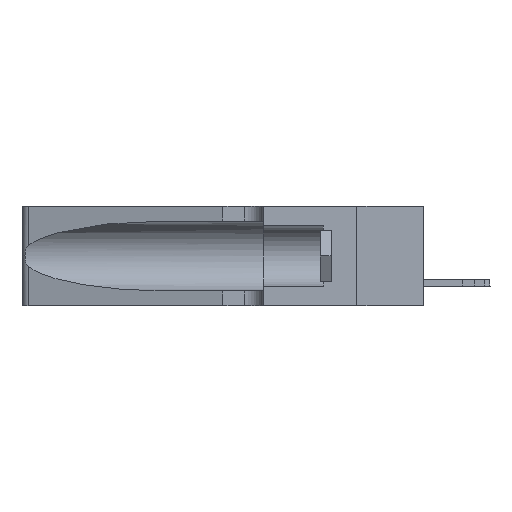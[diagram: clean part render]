
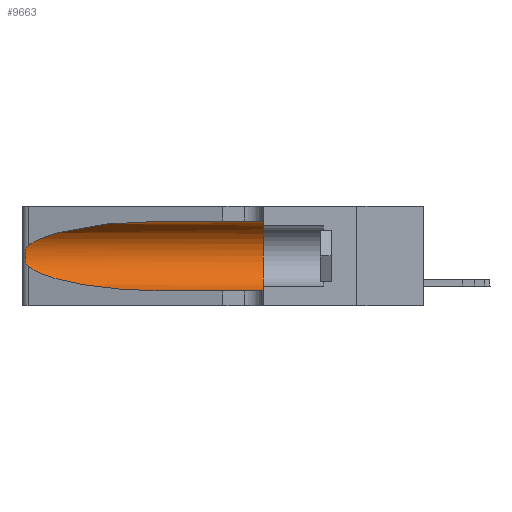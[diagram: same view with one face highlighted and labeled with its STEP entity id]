
A CAD part, left-side view. The second image highlights one B-rep face of the part: STEP entity #9663.
In plain terms, the highlighted cylindrical face has radius 3.308 mm (diameter 6.617 mm), a partial arc.
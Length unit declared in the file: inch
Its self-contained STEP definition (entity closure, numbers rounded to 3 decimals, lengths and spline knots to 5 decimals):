
#384 = LINE ( 'NONE', #15613, #35204 ) ;
#454 = CARTESIAN_POINT ( 'NONE',  ( 0.1305, 0.35, 0.31525 ) ) ;
#845 = VECTOR ( 'NONE', #1334, 39.37008 ) ;
#966 = EDGE_CURVE ( 'NONE', #18151, #34993, #30599, .T. ) ;
#1035 = DIRECTION ( 'NONE',  ( 0., 1., 0. ) ) ;
#1334 = DIRECTION ( 'NONE',  ( 0., -1., 0. ) ) ;
#1512 = FACE_OUTER_BOUND ( 'NONE', #7337, .T. ) ;
#2350 = ORIENTED_EDGE ( 'NONE', *, *, #14464, .T. ) ;
#3958 = AXIS2_PLACEMENT_3D ( 'NONE', #23640, #1035, #27833 ) ;
#4090 = CARTESIAN_POINT ( 'NONE',  ( 0.25487, 1.22718, 0.22369 ) ) ;
#4104 = CARTESIAN_POINT ( 'NONE',  ( 0.1305, 0.72297, 0.31525 ) ) ;
#4166 = DIRECTION ( 'NONE',  ( 0., -1., 0. ) ) ;
#4919 = CARTESIAN_POINT ( 'NONE',  ( 0.18966, 0.96281, 0.31525 ) ) ;
#5788 = VERTEX_POINT ( 'NONE', #4104 ) ;
#6004 = CYLINDRICAL_SURFACE ( 'NONE', #32241, 0.13025 ) ;
#6636 = ORIENTED_EDGE ( 'NONE', *, *, #18487, .T. ) ;
#7226 = CARTESIAN_POINT ( 'NONE',  ( 0.25854, 1.2359, 0.20912 ) ) ;
#7337 = EDGE_LOOP ( 'NONE', ( #6636, #29900, #20356, #2350, #36368, #18727 ) ) ;
#8835 =( BOUNDED_CURVE ( )  B_SPLINE_CURVE ( 3, ( #22195, #4919, #31044, #19324 ),
 .UNSPECIFIED., .F., .T. ) 
 B_SPLINE_CURVE_WITH_KNOTS ( ( 4, 4 ),
 ( 1.5708, 2.84003 ),
 .UNSPECIFIED. ) 
 CURVE ( )  GEOMETRIC_REPRESENTATION_ITEM ( )  RATIONAL_B_SPLINE_CURVE ( ( 1., 0.87, 0.87, 1. ) ) 
 REPRESENTATION_ITEM ( '' )  );
#8963 = VERTEX_POINT ( 'NONE', #28417 ) ;
#9640 = DIRECTION ( 'NONE',  ( 0., -1., 0. ) ) ;
#9663 = ADVANCED_FACE ( 'NONE', ( #1512 ), #6004, .F. ) ;
#10038 = CARTESIAN_POINT ( 'NONE',  ( 0.25787, 1.23484, 0.2124 ) ) ;
#10166 = CARTESIAN_POINT ( 'NONE',  ( 0.25487, 1.22718, 0.14631 ) ) ;
#12433 = CARTESIAN_POINT ( 'NONE',  ( 0.1305, 1.61858, 0.05475 ) ) ;
#12787 = CARTESIAN_POINT ( 'NONE',  ( 0.26075, 1.23896, 0.178 ) ) ;
#12913 = CARTESIAN_POINT ( 'NONE',  ( 0.25639, 1.23186, 0.15144 ) ) ;
#13248 = EDGE_CURVE ( 'NONE', #5788, #20869, #384, .T. ) ;
#14464 = EDGE_CURVE ( 'NONE', #34993, #20847, #26181, .T. ) ;
#15613 = CARTESIAN_POINT ( 'NONE',  ( 0.1305, 1.61858, 0.31525 ) ) ;
#16818 = CARTESIAN_POINT ( 'NONE',  ( 0.1305, 0.72297, 0.05475 ) ) ;
#17436 = CARTESIAN_POINT ( 'NONE',  ( 0.25487, 1.22718, 0.14631 ) ) ;
#18151 = VERTEX_POINT ( 'NONE', #31863 ) ;
#18472 = CARTESIAN_POINT ( 'NONE',  ( 0.26017, 1.23833, 0.17102 ) ) ;
#18487 = EDGE_CURVE ( 'NONE', #5788, #8963, #8835, .T. ) ;
#18727 = ORIENTED_EDGE ( 'NONE', *, *, #13248, .F. ) ;
#19008 = CARTESIAN_POINT ( 'NONE',  ( 0.18966, 0.96281, 0.05475 ) ) ;
#19282 = EDGE_CURVE ( 'NONE', #20869, #20847, #23601, .T. ) ;
#19324 = CARTESIAN_POINT ( 'NONE',  ( 0.25487, 1.22718, 0.22369 ) ) ;
#20356 = ORIENTED_EDGE ( 'NONE', *, *, #966, .T. ) ;
#20686 = EDGE_CURVE ( 'NONE', #8963, #18151, #23356, .T. ) ;
#20847 = VERTEX_POINT ( 'NONE', #27337 ) ;
#20869 = VERTEX_POINT ( 'NONE', #454 ) ;
#21743 = CARTESIAN_POINT ( 'NONE',  ( 0.1305, 0.72297, 0.05475 ) ) ;
#22195 = CARTESIAN_POINT ( 'NONE',  ( 0.1305, 0.72297, 0.31525 ) ) ;
#23356 = B_SPLINE_CURVE_WITH_KNOTS ( 'NONE', 3,
 ( #4090, #33241, #30219, #10038, #7226, #27179, #24541, #12787, #18472, #24256, #32981, #12913, #27438, #10166 ),
 .UNSPECIFIED., .F., .F.,
 ( 4, 2, 2, 2, 2, 2, 4 ),
 ( 0., 0.00027, 0.00053, 0.00107, 0.0016, 0.00187, 0.00214 ),
 .UNSPECIFIED. ) ;
#23601 = CIRCLE ( 'NONE', #3958, 0.13025 ) ;
#23640 = CARTESIAN_POINT ( 'NONE',  ( 0.1305, 0.35, 0.185 ) ) ;
#24256 = CARTESIAN_POINT ( 'NONE',  ( 0.25856, 1.23593, 0.16098 ) ) ;
#24541 = CARTESIAN_POINT ( 'NONE',  ( 0.26075, 1.23896, 0.19203 ) ) ;
#26181 = LINE ( 'NONE', #12433, #845 ) ;
#26792 = CARTESIAN_POINT ( 'NONE',  ( 0.1305, 1.61858, 0.185 ) ) ;
#27179 = CARTESIAN_POINT ( 'NONE',  ( 0.26018, 1.23835, 0.19895 ) ) ;
#27337 = CARTESIAN_POINT ( 'NONE',  ( 0.1305, 0.35, 0.05475 ) ) ;
#27438 = CARTESIAN_POINT ( 'NONE',  ( 0.25555, 1.22993, 0.14849 ) ) ;
#27833 = DIRECTION ( 'NONE',  ( 0., 0., 1. ) ) ;
#28417 = CARTESIAN_POINT ( 'NONE',  ( 0.25487, 1.22718, 0.22369 ) ) ;
#29900 = ORIENTED_EDGE ( 'NONE', *, *, #20686, .T. ) ;
#30219 = CARTESIAN_POINT ( 'NONE',  ( 0.25639, 1.23184, 0.21858 ) ) ;
#30599 =( BOUNDED_CURVE ( )  B_SPLINE_CURVE ( 3, ( #17436, #30734, #19008, #21743 ),
 .UNSPECIFIED., .F., .F. ) 
 B_SPLINE_CURVE_WITH_KNOTS ( ( 4, 4 ),
 ( 3.44316, 4.71239 ),
 .UNSPECIFIED. ) 
 CURVE ( )  GEOMETRIC_REPRESENTATION_ITEM ( )  RATIONAL_B_SPLINE_CURVE ( ( 1., 0.87, 0.87, 1. ) ) 
 REPRESENTATION_ITEM ( '' )  );
#30734 = CARTESIAN_POINT ( 'NONE',  ( 0.2373, 1.15595, 0.08982 ) ) ;
#31044 = CARTESIAN_POINT ( 'NONE',  ( 0.2373, 1.15595, 0.28018 ) ) ;
#31863 = CARTESIAN_POINT ( 'NONE',  ( 0.25487, 1.22718, 0.14631 ) ) ;
#32241 = AXIS2_PLACEMENT_3D ( 'NONE', #26792, #9640, #34538 ) ;
#32981 = CARTESIAN_POINT ( 'NONE',  ( 0.25789, 1.23486, 0.15765 ) ) ;
#33241 = CARTESIAN_POINT ( 'NONE',  ( 0.25555, 1.22994, 0.2215 ) ) ;
#34538 = DIRECTION ( 'NONE',  ( 0., 0., -1. ) ) ;
#34993 = VERTEX_POINT ( 'NONE', #16818 ) ;
#35204 = VECTOR ( 'NONE', #4166, 39.37008 ) ;
#36368 = ORIENTED_EDGE ( 'NONE', *, *, #19282, .F. ) ;
